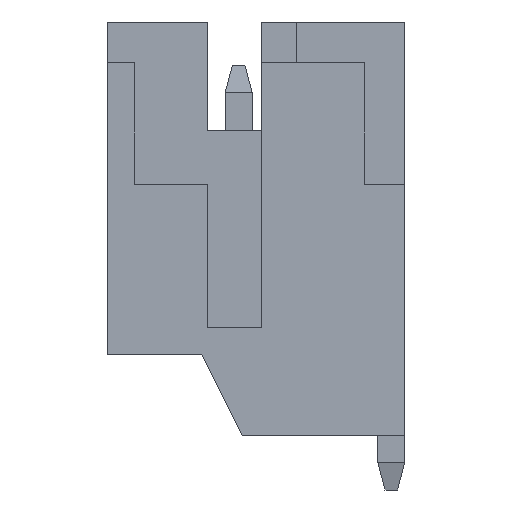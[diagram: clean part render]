
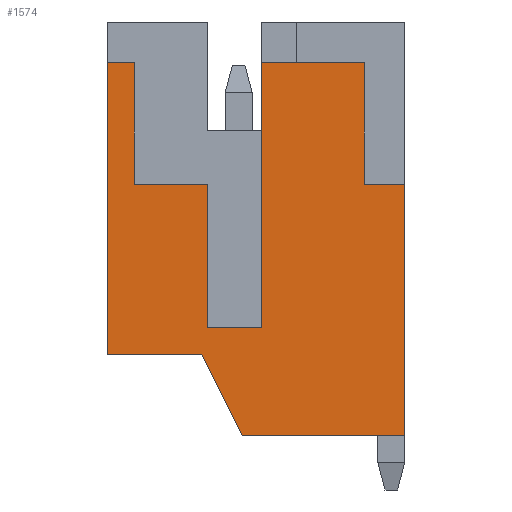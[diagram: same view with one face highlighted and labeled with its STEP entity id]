
A CAD part, left-side view. The second image highlights one B-rep face of the part: STEP entity #1574.
In plain terms, the highlighted planar face has unit normal (-1, 0, 0).
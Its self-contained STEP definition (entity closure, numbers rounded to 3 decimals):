
#122 = VECTOR ( 'NONE', #257, 1000. ) ;
#125 = VERTEX_POINT ( 'NONE', #2610 ) ;
#185 = LINE ( 'NONE', #1106, #6299 ) ;
#257 = DIRECTION ( 'NONE',  ( 0., -0.447, -0.894 ) ) ;
#318 = LINE ( 'NONE', #5441, #6324 ) ;
#371 = CARTESIAN_POINT ( 'NONE',  ( -3., -3.07, 3.15 ) ) ;
#407 = EDGE_CURVE ( 'NONE', #2199, #599, #5813, .T. ) ;
#415 = CARTESIAN_POINT ( 'NONE',  ( -3., -0.42, 3.15 ) ) ;
#557 = CARTESIAN_POINT ( 'NONE',  ( -3., 2.43, 5.4 ) ) ;
#574 = CARTESIAN_POINT ( 'NONE',  ( -3., 2.43, 0. ) ) ;
#599 = VERTEX_POINT ( 'NONE', #371 ) ;
#749 = CARTESIAN_POINT ( 'NONE',  ( -3., 1.93, 3.15 ) ) ;
#822 = CARTESIAN_POINT ( 'NONE',  ( -3., -2.32, 5.4 ) ) ;
#874 = VECTOR ( 'NONE', #1092, 1000. ) ;
#903 = EDGE_CURVE ( 'NONE', #4610, #599, #2597, .T. ) ;
#992 = VECTOR ( 'NONE', #4946, 1000. ) ;
#1053 = ORIENTED_EDGE ( 'NONE', *, *, #5452, .T. ) ;
#1092 = DIRECTION ( 'NONE',  ( 0., 0., 1. ) ) ;
#1106 = CARTESIAN_POINT ( 'NONE',  ( -3., 2.43, 6.15 ) ) ;
#1147 = ORIENTED_EDGE ( 'NONE', *, *, #903, .T. ) ;
#1377 = EDGE_CURVE ( 'NONE', #2989, #125, #7329, .T. ) ;
#1438 = ORIENTED_EDGE ( 'NONE', *, *, #2429, .T. ) ;
#1521 = CARTESIAN_POINT ( 'NONE',  ( -3., 0.58, 3.15 ) ) ;
#1531 = CARTESIAN_POINT ( 'NONE',  ( -3., -3.07, -1.5 ) ) ;
#1560 = ORIENTED_EDGE ( 'NONE', *, *, #7333, .F. ) ;
#1574 = ADVANCED_FACE ( 'NONE', ( #5867 ), #4694, .T. ) ;
#1712 = VECTOR ( 'NONE', #3262, 1000. ) ;
#1718 = CARTESIAN_POINT ( 'NONE',  ( -3., -2.32, 3.15 ) ) ;
#1848 = LINE ( 'NONE', #7243, #122 ) ;
#1884 = LINE ( 'NONE', #6973, #4105 ) ;
#2086 = VERTEX_POINT ( 'NONE', #4663 ) ;
#2199 = VERTEX_POINT ( 'NONE', #6013 ) ;
#2201 = DIRECTION ( 'NONE',  ( 0., -1., 0. ) ) ;
#2292 = ORIENTED_EDGE ( 'NONE', *, *, #5538, .T. ) ;
#2352 = CARTESIAN_POINT ( 'NONE',  ( -3., 0., 0. ) ) ;
#2389 = EDGE_CURVE ( 'NONE', #2199, #6610, #318, .T. ) ;
#2429 = EDGE_CURVE ( 'NONE', #3394, #4137, #1848, .T. ) ;
#2597 = LINE ( 'NONE', #2947, #874 ) ;
#2610 = CARTESIAN_POINT ( 'NONE',  ( -3., -0.42, 0.5 ) ) ;
#2712 = VECTOR ( 'NONE', #2201, 1000. ) ;
#2726 = DIRECTION ( 'NONE',  ( 0., -1., 0. ) ) ;
#2755 = CARTESIAN_POINT ( 'NONE',  ( -3., 0.68, 0. ) ) ;
#2760 = CARTESIAN_POINT ( 'NONE',  ( -3., 1.93, 5.4 ) ) ;
#2947 = CARTESIAN_POINT ( 'NONE',  ( -3., -3.07, 6.15 ) ) ;
#2979 = DIRECTION ( 'NONE',  ( 0., 1., 0. ) ) ;
#2989 = VERTEX_POINT ( 'NONE', #5976 ) ;
#3006 = DIRECTION ( 'NONE',  ( 0., -1., 0. ) ) ;
#3088 = ORIENTED_EDGE ( 'NONE', *, *, #2389, .T. ) ;
#3262 = DIRECTION ( 'NONE',  ( 0., 0., -1. ) ) ;
#3394 = VERTEX_POINT ( 'NONE', #2755 ) ;
#3519 = VERTEX_POINT ( 'NONE', #749 ) ;
#3547 = LINE ( 'NONE', #1521, #1712 ) ;
#3555 = DIRECTION ( 'NONE',  ( -1., 0., 0. ) ) ;
#3724 = LINE ( 'NONE', #415, #992 ) ;
#3730 = LINE ( 'NONE', #6806, #7005 ) ;
#3774 = ORIENTED_EDGE ( 'NONE', *, *, #1377, .T. ) ;
#3894 = VERTEX_POINT ( 'NONE', #557 ) ;
#3897 = AXIS2_PLACEMENT_3D ( 'NONE', #2352, #3555, #6951 ) ;
#3998 = VECTOR ( 'NONE', #7406, 1000. ) ;
#4082 = VECTOR ( 'NONE', #6678, 1000. ) ;
#4105 = VECTOR ( 'NONE', #2979, 1000. ) ;
#4137 = VERTEX_POINT ( 'NONE', #6917 ) ;
#4536 = LINE ( 'NONE', #5144, #3998 ) ;
#4554 = LINE ( 'NONE', #6476, #7092 ) ;
#4587 = ORIENTED_EDGE ( 'NONE', *, *, #407, .F. ) ;
#4610 = VERTEX_POINT ( 'NONE', #4888 ) ;
#4663 = CARTESIAN_POINT ( 'NONE',  ( -3., 0.58, 0.5 ) ) ;
#4670 = DIRECTION ( 'NONE',  ( 0., 0., -1. ) ) ;
#4694 = PLANE ( 'NONE',  #3897 ) ;
#4731 = EDGE_CURVE ( 'NONE', #3519, #7513, #3730, .T. ) ;
#4789 = ORIENTED_EDGE ( 'NONE', *, *, #5176, .F. ) ;
#4888 = CARTESIAN_POINT ( 'NONE',  ( -3., -3.07, -1.5 ) ) ;
#4946 = DIRECTION ( 'NONE',  ( 0., -1., 0. ) ) ;
#5012 = CARTESIAN_POINT ( 'NONE',  ( -3., -0.42, 6.15 ) ) ;
#5144 = CARTESIAN_POINT ( 'NONE',  ( -3., -3.07, 5.4 ) ) ;
#5149 = EDGE_CURVE ( 'NONE', #4137, #4610, #6092, .T. ) ;
#5176 = EDGE_CURVE ( 'NONE', #3519, #6274, #3724, .T. ) ;
#5195 = DIRECTION ( 'NONE',  ( 0., -1., 0. ) ) ;
#5275 = VECTOR ( 'NONE', #2726, 1000. ) ;
#5296 = ORIENTED_EDGE ( 'NONE', *, *, #4731, .T. ) ;
#5385 = VERTEX_POINT ( 'NONE', #574 ) ;
#5418 = ORIENTED_EDGE ( 'NONE', *, *, #7122, .T. ) ;
#5441 = CARTESIAN_POINT ( 'NONE',  ( -3., -2.32, 3.15 ) ) ;
#5452 = EDGE_CURVE ( 'NONE', #6610, #2989, #1884, .T. ) ;
#5467 = DIRECTION ( 'NONE',  ( 0., 0., 1. ) ) ;
#5538 = EDGE_CURVE ( 'NONE', #7513, #3894, #4536, .T. ) ;
#5620 = DIRECTION ( 'NONE',  ( 0., 0., 1. ) ) ;
#5665 = CARTESIAN_POINT ( 'NONE',  ( -3., -0.42, 0.5 ) ) ;
#5712 = EDGE_CURVE ( 'NONE', #2086, #125, #5817, .T. ) ;
#5813 = LINE ( 'NONE', #1718, #5985 ) ;
#5817 = LINE ( 'NONE', #5665, #2712 ) ;
#5850 = EDGE_CURVE ( 'NONE', #3894, #5385, #185, .T. ) ;
#5867 = FACE_OUTER_BOUND ( 'NONE', #7078, .T. ) ;
#5976 = CARTESIAN_POINT ( 'NONE',  ( -3., -0.42, 5.4 ) ) ;
#5985 = VECTOR ( 'NONE', #5195, 1000. ) ;
#6013 = CARTESIAN_POINT ( 'NONE',  ( -3., -2.32, 3.15 ) ) ;
#6092 = LINE ( 'NONE', #1531, #5275 ) ;
#6274 = VERTEX_POINT ( 'NONE', #6330 ) ;
#6299 = VECTOR ( 'NONE', #4670, 1000. ) ;
#6324 = VECTOR ( 'NONE', #5467, 1000. ) ;
#6330 = CARTESIAN_POINT ( 'NONE',  ( -3., 0.58, 3.15 ) ) ;
#6335 = ORIENTED_EDGE ( 'NONE', *, *, #5712, .F. ) ;
#6429 = ORIENTED_EDGE ( 'NONE', *, *, #5850, .T. ) ;
#6476 = CARTESIAN_POINT ( 'NONE',  ( -3., 2.43, 0. ) ) ;
#6610 = VERTEX_POINT ( 'NONE', #822 ) ;
#6678 = DIRECTION ( 'NONE',  ( 0., 0., -1. ) ) ;
#6806 = CARTESIAN_POINT ( 'NONE',  ( -3., 1.93, 3.15 ) ) ;
#6917 = CARTESIAN_POINT ( 'NONE',  ( -3., -0.07, -1.5 ) ) ;
#6951 = DIRECTION ( 'NONE',  ( 0., -1., 0. ) ) ;
#6973 = CARTESIAN_POINT ( 'NONE',  ( -3., -3.07, 5.4 ) ) ;
#7005 = VECTOR ( 'NONE', #5620, 1000. ) ;
#7051 = ORIENTED_EDGE ( 'NONE', *, *, #5149, .T. ) ;
#7078 = EDGE_LOOP ( 'NONE', ( #2292, #6429, #5418, #1438, #7051, #1147, #4587, #3088, #1053, #3774, #6335, #1560, #4789, #5296 ) ) ;
#7092 = VECTOR ( 'NONE', #3006, 1000. ) ;
#7122 = EDGE_CURVE ( 'NONE', #5385, #3394, #4554, .T. ) ;
#7243 = CARTESIAN_POINT ( 'NONE',  ( -3., -0.07, -1.5 ) ) ;
#7329 = LINE ( 'NONE', #5012, #4082 ) ;
#7333 = EDGE_CURVE ( 'NONE', #6274, #2086, #3547, .T. ) ;
#7406 = DIRECTION ( 'NONE',  ( 0., 1., 0. ) ) ;
#7513 = VERTEX_POINT ( 'NONE', #2760 ) ;
